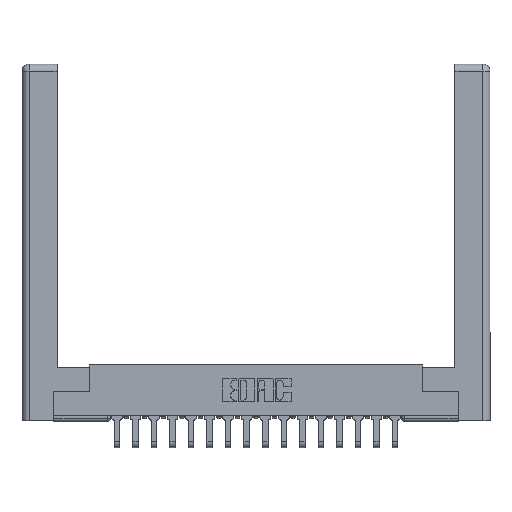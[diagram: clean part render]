
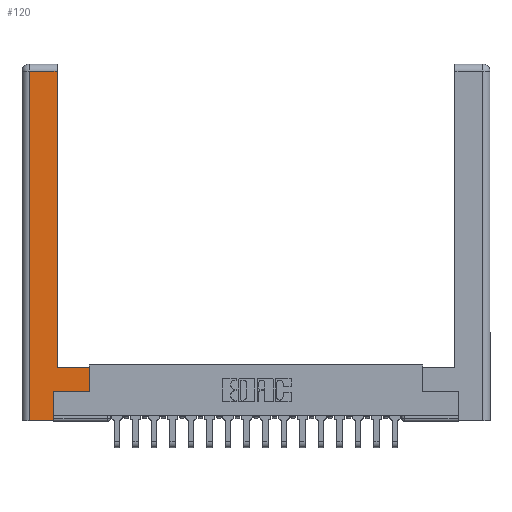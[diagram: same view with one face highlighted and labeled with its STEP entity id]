
A CAD part, top view. The second image highlights one B-rep face of the part: STEP entity #120.
In plain terms, the highlighted planar face has unit normal (0, 0, 1).
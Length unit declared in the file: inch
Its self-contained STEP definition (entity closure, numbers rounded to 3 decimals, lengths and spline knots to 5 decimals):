
#120 = ADVANCED_FACE ( 'NONE', ( #17372 ), #18909, .F. ) ;
#518 = VECTOR ( 'NONE', #17479, 39.37008 ) ;
#611 = VERTEX_POINT ( 'NONE', #9236 ) ;
#728 = VERTEX_POINT ( 'NONE', #11389 ) ;
#1191 = DIRECTION ( 'NONE',  ( -1., 0., 0. ) ) ;
#2147 = VERTEX_POINT ( 'NONE', #3467 ) ;
#2200 = DIRECTION ( 'NONE',  ( 0., 1., 0. ) ) ;
#2726 = ORIENTED_EDGE ( 'NONE', *, *, #8440, .T. ) ;
#3467 = CARTESIAN_POINT ( 'NONE',  ( 0.0615, 0., 0. ) ) ;
#4699 = VECTOR ( 'NONE', #2200, 39.37008 ) ;
#5143 = EDGE_CURVE ( 'NONE', #728, #10892, #12753, .T. ) ;
#5574 = CARTESIAN_POINT ( 'NONE',  ( 0.295, 2.94, 0. ) ) ;
#5664 = CARTESIAN_POINT ( 'NONE',  ( 0.565, 0.45, 0. ) ) ;
#6033 = AXIS2_PLACEMENT_3D ( 'NONE', #8947, #20752, #7530 ) ;
#6264 = VECTOR ( 'NONE', #1191, 39.37008 ) ;
#7287 = EDGE_CURVE ( 'NONE', #7607, #20420, #14570, .T. ) ;
#7318 = CARTESIAN_POINT ( 'NONE',  ( 0.295, 3., 0. ) ) ;
#7530 = DIRECTION ( 'NONE',  ( -1., 0., 0. ) ) ;
#7607 = VERTEX_POINT ( 'NONE', #5574 ) ;
#7909 = EDGE_CURVE ( 'NONE', #10029, #611, #13193, .T. ) ;
#8086 = CARTESIAN_POINT ( 'NONE',  ( 0.265, 0.245, 0. ) ) ;
#8440 = EDGE_CURVE ( 'NONE', #611, #728, #18780, .T. ) ;
#8947 = CARTESIAN_POINT ( 'NONE',  ( 0., 0., 0. ) ) ;
#9236 = CARTESIAN_POINT ( 'NONE',  ( 0.565, 0.245, 0. ) ) ;
#9412 = LINE ( 'NONE', #15625, #20375 ) ;
#10029 = VERTEX_POINT ( 'NONE', #8086 ) ;
#10081 = VECTOR ( 'NONE', #19425, 39.37008 ) ;
#10088 = CARTESIAN_POINT ( 'NONE',  ( 0.265, 0., 0. ) ) ;
#10683 = VECTOR ( 'NONE', #20497, 39.37008 ) ;
#10892 = VERTEX_POINT ( 'NONE', #14452 ) ;
#11270 = ORIENTED_EDGE ( 'NONE', *, *, #13859, .T. ) ;
#11372 = ORIENTED_EDGE ( 'NONE', *, *, #5143, .T. ) ;
#11389 = CARTESIAN_POINT ( 'NONE',  ( 0.565, 0.45, 0. ) ) ;
#11778 = EDGE_CURVE ( 'NONE', #10892, #7607, #17264, .T. ) ;
#12320 = DIRECTION ( 'NONE',  ( 0., 1., 0. ) ) ;
#12620 = VERTEX_POINT ( 'NONE', #10088 ) ;
#12654 = ORIENTED_EDGE ( 'NONE', *, *, #17689, .T. ) ;
#12753 = LINE ( 'NONE', #14184, #10081 ) ;
#12781 = EDGE_LOOP ( 'NONE', ( #14512, #20307, #17825, #12654, #11270, #17163, #2726, #11372 ) ) ;
#13193 = LINE ( 'NONE', #20190, #18153 ) ;
#13384 = EDGE_CURVE ( 'NONE', #20420, #2147, #9412, .T. ) ;
#13500 = LINE ( 'NONE', #17114, #10683 ) ;
#13859 = EDGE_CURVE ( 'NONE', #12620, #10029, #17571, .T. ) ;
#14184 = CARTESIAN_POINT ( 'NONE',  ( 0.295, 0.45, 0. ) ) ;
#14452 = CARTESIAN_POINT ( 'NONE',  ( 0.295, 0.45, 0. ) ) ;
#14512 = ORIENTED_EDGE ( 'NONE', *, *, #11778, .T. ) ;
#14570 = LINE ( 'NONE', #17971, #6264 ) ;
#15491 = CARTESIAN_POINT ( 'NONE',  ( 0.0615, 2.94, 0. ) ) ;
#15625 = CARTESIAN_POINT ( 'NONE',  ( 0.0615, 0., 0. ) ) ;
#16066 = DIRECTION ( 'NONE',  ( 0., -1., 0. ) ) ;
#17114 = CARTESIAN_POINT ( 'NONE',  ( 0.265, 0., 0. ) ) ;
#17141 = CARTESIAN_POINT ( 'NONE',  ( 0.265, 0.245, 0. ) ) ;
#17163 = ORIENTED_EDGE ( 'NONE', *, *, #7909, .T. ) ;
#17264 = LINE ( 'NONE', #7318, #518 ) ;
#17372 = FACE_OUTER_BOUND ( 'NONE', #12781, .T. ) ;
#17479 = DIRECTION ( 'NONE',  ( 0., 1., 0. ) ) ;
#17571 = LINE ( 'NONE', #17141, #4699 ) ;
#17689 = EDGE_CURVE ( 'NONE', #2147, #12620, #13500, .T. ) ;
#17825 = ORIENTED_EDGE ( 'NONE', *, *, #13384, .T. ) ;
#17971 = CARTESIAN_POINT ( 'NONE',  ( 0.0615, 2.94, 0. ) ) ;
#18153 = VECTOR ( 'NONE', #19971, 39.37008 ) ;
#18532 = VECTOR ( 'NONE', #12320, 39.37008 ) ;
#18780 = LINE ( 'NONE', #5664, #18532 ) ;
#18909 = PLANE ( 'NONE',  #6033 ) ;
#19425 = DIRECTION ( 'NONE',  ( -1., 0., 0. ) ) ;
#19971 = DIRECTION ( 'NONE',  ( 1., 0., 0. ) ) ;
#20190 = CARTESIAN_POINT ( 'NONE',  ( 0.565, 0.245, 0. ) ) ;
#20307 = ORIENTED_EDGE ( 'NONE', *, *, #7287, .T. ) ;
#20375 = VECTOR ( 'NONE', #16066, 39.37008 ) ;
#20420 = VERTEX_POINT ( 'NONE', #15491 ) ;
#20497 = DIRECTION ( 'NONE',  ( 1., 0., 0. ) ) ;
#20752 = DIRECTION ( 'NONE',  ( 0., 0., -1. ) ) ;
